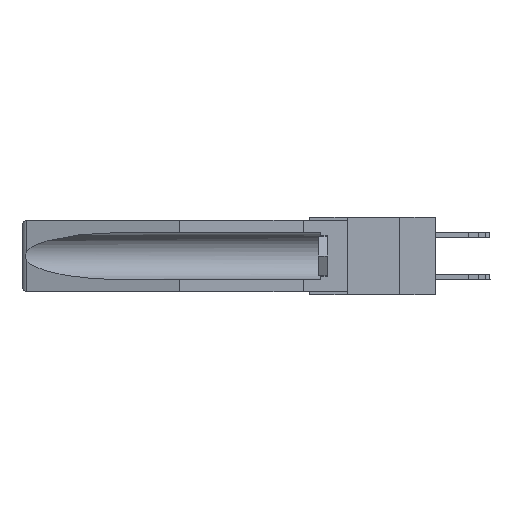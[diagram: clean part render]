
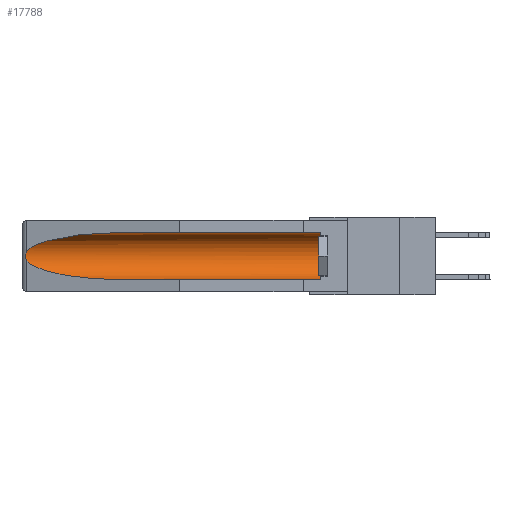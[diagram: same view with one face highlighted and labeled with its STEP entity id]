
A CAD part, left-side view. The second image highlights one B-rep face of the part: STEP entity #17788.
In plain terms, the highlighted cylindrical face has radius 2.857 mm (diameter 5.715 mm), a partial arc.
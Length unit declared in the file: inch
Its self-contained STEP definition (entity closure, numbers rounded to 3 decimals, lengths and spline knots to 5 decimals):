
#12 = CARTESIAN_POINT ( 'NONE',  ( 0.155, 0.126, -0.059 ) ) ;
#190 = DIRECTION ( 'NONE',  ( 0., 0., 1. ) ) ;
#339 = CYLINDRICAL_SURFACE ( 'NONE', #7580, 0.1125 ) ;
#981 = DIRECTION ( 'NONE',  ( 0., 1., 0. ) ) ;
#1857 = CARTESIAN_POINT ( 'NONE',  ( 0.26597, 1.52961, -0.15275 ) ) ;
#2834 =( BOUNDED_CURVE ( )  B_SPLINE_CURVE ( 3, ( #14953, #18621, #16881, #22142 ),
 .UNSPECIFIED., .F., .T. ) 
 B_SPLINE_CURVE_WITH_KNOTS ( ( 4, 4 ),
 ( 4.71239, 6.08839 ),
 .UNSPECIFIED. ) 
 CURVE ( )  GEOMETRIC_REPRESENTATION_ITEM ( )  RATIONAL_B_SPLINE_CURVE ( ( 1., 0.848, 0.848, 1. ) ) 
 REPRESENTATION_ITEM ( '' )  );
#2923 = LINE ( 'NONE', #20548, #17022 ) ;
#3093 = ORIENTED_EDGE ( 'NONE', *, *, #5619, .T. ) ;
#3115 = VECTOR ( 'NONE', #14161, 39.37008 ) ;
#3419 = ORIENTED_EDGE ( 'NONE', *, *, #21024, .T. ) ;
#3605 = CARTESIAN_POINT ( 'NONE',  ( 0.155, -0.30754, -0.1715 ) ) ;
#3672 = CARTESIAN_POINT ( 'NONE',  ( 0.155, 1.07973, -0.284 ) ) ;
#3763 = VERTEX_POINT ( 'NONE', #9635 ) ;
#3832 = EDGE_LOOP ( 'NONE', ( #11440, #3419, #9149, #20149, #3093, #19486 ) ) ;
#3899 = CARTESIAN_POINT ( 'NONE',  ( 0.155, 1.07973, -0.284 ) ) ;
#4285 = VERTEX_POINT ( 'NONE', #12 ) ;
#4548 = EDGE_CURVE ( 'NONE', #3763, #21469, #2834, .T. ) ;
#5425 = CARTESIAN_POINT ( 'NONE',  ( 0.2673, 1.5327, -0.16383 ) ) ;
#5492 = CARTESIAN_POINT ( 'NONE',  ( 0.26537, 1.52718, -0.19328 ) ) ;
#5619 = EDGE_CURVE ( 'NONE', #9444, #4285, #6191, .T. ) ;
#5683 = CARTESIAN_POINT ( 'NONE',  ( 0.25451, 1.48313, -0.24835 ) ) ;
#5899 = LINE ( 'NONE', #19179, #3115 ) ;
#6083 = CARTESIAN_POINT ( 'NONE',  ( 0.155, 0.126, -0.284 ) ) ;
#6191 = CIRCLE ( 'NONE', #9935, 0.1125 ) ;
#7580 = AXIS2_PLACEMENT_3D ( 'NONE', #3605, #19500, #190 ) ;
#7650 =( BOUNDED_CURVE ( )  B_SPLINE_CURVE ( 3, ( #10997, #5683, #14483, #3899 ),
 .UNSPECIFIED., .F., .F. ) 
 B_SPLINE_CURVE_WITH_KNOTS ( ( 4, 4 ),
 ( 0.1948, 1.5708 ),
 .UNSPECIFIED. ) 
 CURVE ( )  GEOMETRIC_REPRESENTATION_ITEM ( )  RATIONAL_B_SPLINE_CURVE ( ( 1., 0.848, 0.848, 1. ) ) 
 REPRESENTATION_ITEM ( '' )  );
#8065 = VERTEX_POINT ( 'NONE', #3672 ) ;
#8156 = EDGE_CURVE ( 'NONE', #18689, #8065, #7650, .T. ) ;
#8869 = CARTESIAN_POINT ( 'NONE',  ( 0.2675, 1.53308, -0.16763 ) ) ;
#8948 = CARTESIAN_POINT ( 'NONE',  ( 0.2673, 1.53269, -0.17917 ) ) ;
#9149 = ORIENTED_EDGE ( 'NONE', *, *, #8156, .T. ) ;
#9444 = VERTEX_POINT ( 'NONE', #6083 ) ;
#9635 = CARTESIAN_POINT ( 'NONE',  ( 0.155, 1.07973, -0.059 ) ) ;
#9935 = AXIS2_PLACEMENT_3D ( 'NONE', #15706, #17490, #19241 ) ;
#10351 = EDGE_CURVE ( 'NONE', #9444, #8065, #2923, .T. ) ;
#10997 = CARTESIAN_POINT ( 'NONE',  ( 0.26537, 1.52718, -0.19328 ) ) ;
#11440 = ORIENTED_EDGE ( 'NONE', *, *, #4548, .T. ) ;
#14161 = DIRECTION ( 'NONE',  ( 0., 1., 0. ) ) ;
#14279 = CARTESIAN_POINT ( 'NONE',  ( 0.26597, 1.5296, -0.19026 ) ) ;
#14483 = CARTESIAN_POINT ( 'NONE',  ( 0.21114, 1.30732, -0.284 ) ) ;
#14558 = EDGE_CURVE ( 'NONE', #4285, #3763, #5899, .T. ) ;
#14953 = CARTESIAN_POINT ( 'NONE',  ( 0.155, 1.07973, -0.059 ) ) ;
#14995 = FACE_OUTER_BOUND ( 'NONE', #3832, .T. ) ;
#15281 = CARTESIAN_POINT ( 'NONE',  ( 0.26537, 1.52718, -0.14972 ) ) ;
#15706 = CARTESIAN_POINT ( 'NONE',  ( 0.155, 0.126, -0.1715 ) ) ;
#16881 = CARTESIAN_POINT ( 'NONE',  ( 0.25451, 1.48313, -0.09465 ) ) ;
#17022 = VECTOR ( 'NONE', #981, 39.37008 ) ;
#17463 = CARTESIAN_POINT ( 'NONE',  ( 0.26655, 1.53094, -0.18657 ) ) ;
#17490 = DIRECTION ( 'NONE',  ( 0., -1., 0. ) ) ;
#17547 = CARTESIAN_POINT ( 'NONE',  ( 0.2675, 1.53308, -0.17534 ) ) ;
#17687 = B_SPLINE_CURVE_WITH_KNOTS ( 'NONE', 3,
 ( #20898, #1857, #21131, #5425, #8869, #17547, #8948, #17463, #14279, #18139 ),
 .UNSPECIFIED., .F., .F.,
 ( 4, 2, 2, 2, 4 ),
 ( 0., 0.00029, 0.00058, 0.00087, 0.00117 ),
 .UNSPECIFIED. ) ;
#17788 = ADVANCED_FACE ( 'NONE', ( #14995 ), #339, .F. ) ;
#18139 = CARTESIAN_POINT ( 'NONE',  ( 0.26537, 1.52718, -0.19328 ) ) ;
#18621 = CARTESIAN_POINT ( 'NONE',  ( 0.21114, 1.30732, -0.059 ) ) ;
#18689 = VERTEX_POINT ( 'NONE', #5492 ) ;
#19179 = CARTESIAN_POINT ( 'NONE',  ( 0.155, -0.30754, -0.059 ) ) ;
#19241 = DIRECTION ( 'NONE',  ( 0., 0., 1. ) ) ;
#19486 = ORIENTED_EDGE ( 'NONE', *, *, #14558, .T. ) ;
#19500 = DIRECTION ( 'NONE',  ( 0., 1., 0. ) ) ;
#20149 = ORIENTED_EDGE ( 'NONE', *, *, #10351, .F. ) ;
#20548 = CARTESIAN_POINT ( 'NONE',  ( 0.155, -0.30754, -0.284 ) ) ;
#20898 = CARTESIAN_POINT ( 'NONE',  ( 0.26537, 1.52718, -0.14972 ) ) ;
#21024 = EDGE_CURVE ( 'NONE', #21469, #18689, #17687, .T. ) ;
#21131 = CARTESIAN_POINT ( 'NONE',  ( 0.26654, 1.53092, -0.15636 ) ) ;
#21469 = VERTEX_POINT ( 'NONE', #15281 ) ;
#22142 = CARTESIAN_POINT ( 'NONE',  ( 0.26537, 1.52718, -0.14972 ) ) ;
